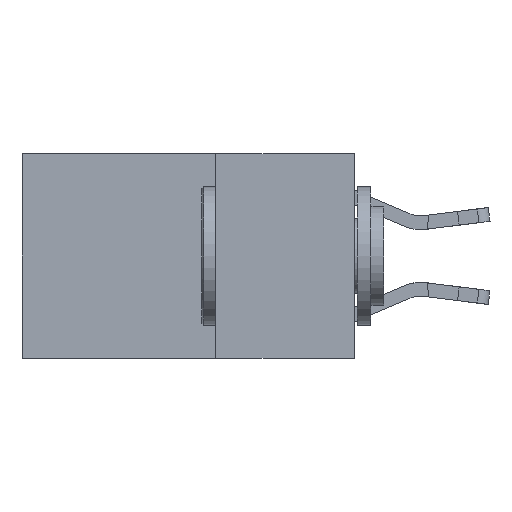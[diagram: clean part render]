
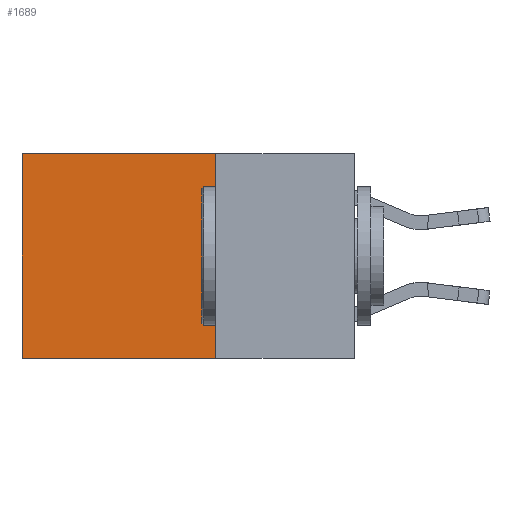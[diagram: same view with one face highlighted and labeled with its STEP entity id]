
A CAD part, left-side view. The second image highlights one B-rep face of the part: STEP entity #1689.
In plain terms, the highlighted planar face has unit normal (-1, 0, 0).
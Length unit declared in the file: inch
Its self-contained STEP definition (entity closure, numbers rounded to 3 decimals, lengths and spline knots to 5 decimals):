
#1382 = EDGE_CURVE ( 'NONE', #11529, #8039, #7977, .T. ) ;
#1689 = ADVANCED_FACE ( 'NONE', ( #7449 ), #2053, .F. ) ;
#1816 = DIRECTION ( 'NONE',  ( 0., 0., -1. ) ) ;
#1958 = DIRECTION ( 'NONE',  ( 1., 0., 0. ) ) ;
#2053 = PLANE ( 'NONE',  #2605 ) ;
#2238 = CARTESIAN_POINT ( 'NONE',  ( 0.2625, 0.25, 0. ) ) ;
#2369 = CARTESIAN_POINT ( 'NONE',  ( 0.2625, 0.6, -0.37 ) ) ;
#2605 = AXIS2_PLACEMENT_3D ( 'NONE', #2238, #1958, #1816 ) ;
#3794 = VECTOR ( 'NONE', #6748, 39.37008 ) ;
#5006 = VECTOR ( 'NONE', #12483, 39.37008 ) ;
#6748 = DIRECTION ( 'NONE',  ( 0., 0., -1. ) ) ;
#7449 = FACE_OUTER_BOUND ( 'NONE', #7507, .T. ) ;
#7501 = ORIENTED_EDGE ( 'NONE', *, *, #8047, .T. ) ;
#7507 = EDGE_LOOP ( 'NONE', ( #7501, #8600, #9170, #14088 ) ) ;
#7724 = EDGE_CURVE ( 'NONE', #11529, #12833, #13197, .T. ) ;
#7802 = CARTESIAN_POINT ( 'NONE',  ( 0.2625, 0.6, 0. ) ) ;
#7977 = LINE ( 'NONE', #12383, #5006 ) ;
#8039 = VERTEX_POINT ( 'NONE', #7802 ) ;
#8047 = EDGE_CURVE ( 'NONE', #8039, #9407, #9747, .T. ) ;
#8048 = CARTESIAN_POINT ( 'NONE',  ( 0.2625, 0.25, -0.37 ) ) ;
#8172 = EDGE_CURVE ( 'NONE', #12833, #9407, #8333, .T. ) ;
#8333 = LINE ( 'NONE', #8048, #13539 ) ;
#8600 = ORIENTED_EDGE ( 'NONE', *, *, #8172, .F. ) ;
#9160 = DIRECTION ( 'NONE',  ( 0., 1., 0. ) ) ;
#9170 = ORIENTED_EDGE ( 'NONE', *, *, #7724, .F. ) ;
#9407 = VERTEX_POINT ( 'NONE', #2369 ) ;
#9747 = LINE ( 'NONE', #14402, #3794 ) ;
#10272 = VECTOR ( 'NONE', #12804, 39.37008 ) ;
#11116 = CARTESIAN_POINT ( 'NONE',  ( 0.2625, 0.25, -0.37 ) ) ;
#11529 = VERTEX_POINT ( 'NONE', #13869 ) ;
#12383 = CARTESIAN_POINT ( 'NONE',  ( 0.2625, 0.25, 0. ) ) ;
#12483 = DIRECTION ( 'NONE',  ( 0., 1., 0. ) ) ;
#12756 = CARTESIAN_POINT ( 'NONE',  ( 0.2625, 0.25, 0. ) ) ;
#12804 = DIRECTION ( 'NONE',  ( 0., 0., -1. ) ) ;
#12833 = VERTEX_POINT ( 'NONE', #11116 ) ;
#13197 = LINE ( 'NONE', #12756, #10272 ) ;
#13539 = VECTOR ( 'NONE', #9160, 39.37008 ) ;
#13869 = CARTESIAN_POINT ( 'NONE',  ( 0.2625, 0.25, 0. ) ) ;
#14088 = ORIENTED_EDGE ( 'NONE', *, *, #1382, .T. ) ;
#14402 = CARTESIAN_POINT ( 'NONE',  ( 0.2625, 0.6, 0. ) ) ;
